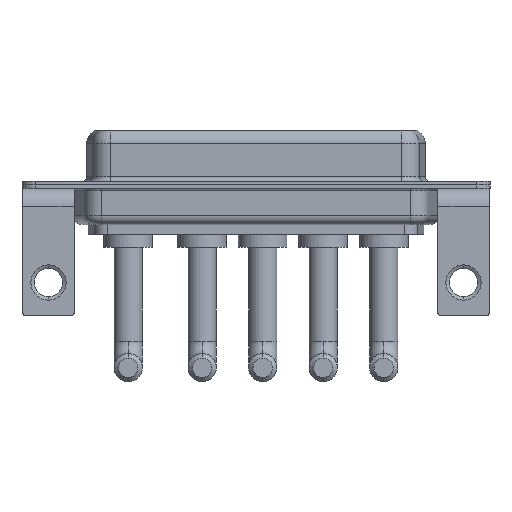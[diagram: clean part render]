
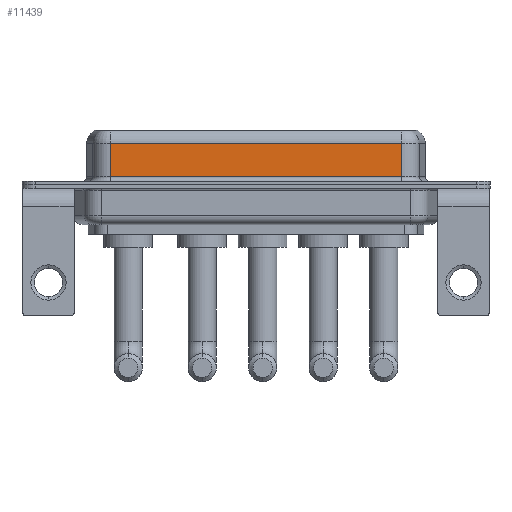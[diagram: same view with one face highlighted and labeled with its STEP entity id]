
A CAD part, front view. The second image highlights one B-rep face of the part: STEP entity #11439.
In plain terms, the highlighted planar face has unit normal (0, -1, 0).
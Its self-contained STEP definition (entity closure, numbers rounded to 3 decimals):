
#168 = VECTOR ( 'NONE', #12945, 1000. ) ;
#257 = VECTOR ( 'NONE', #537, 1000. ) ;
#444 = ORIENTED_EDGE ( 'NONE', *, *, #11603, .T. ) ;
#476 = DIRECTION ( 'NONE',  ( 0., 1., 0. ) ) ;
#537 = DIRECTION ( 'NONE',  ( 0., 0., -1. ) ) ;
#909 = CARTESIAN_POINT ( 'NONE',  ( 7.013, -3.95, 0.9 ) ) ;
#1408 = ORIENTED_EDGE ( 'NONE', *, *, #2203, .T. ) ;
#1413 = CARTESIAN_POINT ( 'NONE',  ( 40.037, -3.95, 4.65 ) ) ;
#1538 = DIRECTION ( 'NONE',  ( 0., 0., -1. ) ) ;
#2203 = EDGE_CURVE ( 'NONE', #3110, #12008, #10889, .T. ) ;
#2484 = LINE ( 'NONE', #11774, #168 ) ;
#2589 = VECTOR ( 'NONE', #1538, 1000. ) ;
#2826 = CARTESIAN_POINT ( 'NONE',  ( 40.037, -3.95, 0.9 ) ) ;
#3110 = VERTEX_POINT ( 'NONE', #7696 ) ;
#3392 = CARTESIAN_POINT ( 'NONE',  ( 40.037, -3.95, 6.4 ) ) ;
#5118 = LINE ( 'NONE', #8250, #10704 ) ;
#6201 = DIRECTION ( 'NONE',  ( 1., 0., 0. ) ) ;
#6684 = PLANE ( 'NONE',  #7810 ) ;
#6859 = CARTESIAN_POINT ( 'NONE',  ( 7.013, -3.95, 6.4 ) ) ;
#7098 = ORIENTED_EDGE ( 'NONE', *, *, #12789, .T. ) ;
#7696 = CARTESIAN_POINT ( 'NONE',  ( 7.013, -3.95, 4.65 ) ) ;
#7810 = AXIS2_PLACEMENT_3D ( 'NONE', #3392, #476, #8586 ) ;
#8250 = CARTESIAN_POINT ( 'NONE',  ( 40.037, -3.95, 0.9 ) ) ;
#8586 = DIRECTION ( 'NONE',  ( 0., 0., 1. ) ) ;
#8733 = VERTEX_POINT ( 'NONE', #1413 ) ;
#10032 = EDGE_LOOP ( 'NONE', ( #12114, #444, #1408, #7098 ) ) ;
#10700 = FACE_OUTER_BOUND ( 'NONE', #10032, .T. ) ;
#10704 = VECTOR ( 'NONE', #6201, 1000. ) ;
#10889 = LINE ( 'NONE', #6859, #2589 ) ;
#10909 = VERTEX_POINT ( 'NONE', #2826 ) ;
#10922 = LINE ( 'NONE', #12967, #257 ) ;
#11439 = ADVANCED_FACE ( 'NONE', ( #10700 ), #6684, .F. ) ;
#11603 = EDGE_CURVE ( 'NONE', #8733, #3110, #2484, .T. ) ;
#11774 = CARTESIAN_POINT ( 'NONE',  ( 40.037, -3.95, 4.65 ) ) ;
#12008 = VERTEX_POINT ( 'NONE', #909 ) ;
#12114 = ORIENTED_EDGE ( 'NONE', *, *, #13160, .F. ) ;
#12789 = EDGE_CURVE ( 'NONE', #12008, #10909, #5118, .T. ) ;
#12945 = DIRECTION ( 'NONE',  ( -1., 0., 0. ) ) ;
#12967 = CARTESIAN_POINT ( 'NONE',  ( 40.037, -3.95, 6.4 ) ) ;
#13160 = EDGE_CURVE ( 'NONE', #8733, #10909, #10922, .T. ) ;
